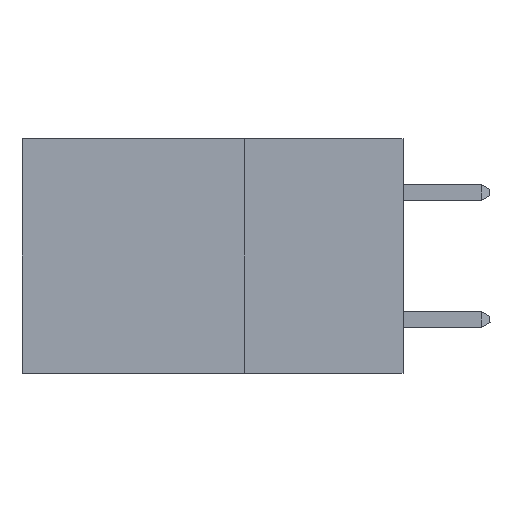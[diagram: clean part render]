
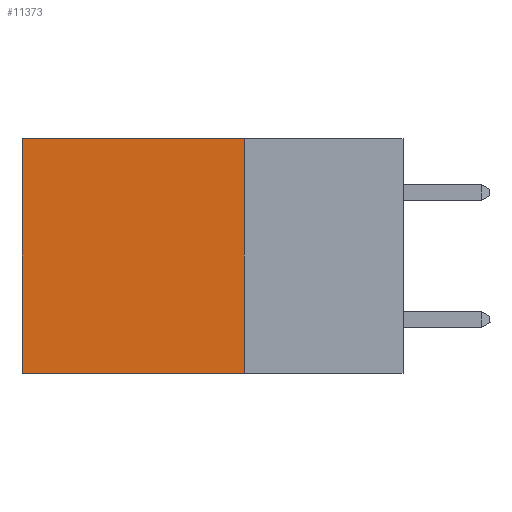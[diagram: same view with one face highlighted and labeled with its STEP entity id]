
A CAD part, left-side view. The second image highlights one B-rep face of the part: STEP entity #11373.
In plain terms, the highlighted planar face has unit normal (-1, 0, 0).
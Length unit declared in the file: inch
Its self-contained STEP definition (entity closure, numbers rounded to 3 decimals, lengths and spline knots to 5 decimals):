
#392 = CARTESIAN_POINT ( 'NONE',  ( 0.2875, 0.25, 0. ) ) ;
#699 = CARTESIAN_POINT ( 'NONE',  ( 0.2875, 0.25, -0.37 ) ) ;
#1184 = VECTOR ( 'NONE', #15054, 39.37008 ) ;
#1190 = CARTESIAN_POINT ( 'NONE',  ( 0.2875, 0.25, 0. ) ) ;
#1632 = LINE ( 'NONE', #13678, #1184 ) ;
#1925 = DIRECTION ( 'NONE',  ( 0., 0., -1. ) ) ;
#1986 = VECTOR ( 'NONE', #7826, 39.37008 ) ;
#1997 = CARTESIAN_POINT ( 'NONE',  ( 0.2875, 0.6, 0. ) ) ;
#2085 = CARTESIAN_POINT ( 'NONE',  ( 0.2875, 0.6, 0. ) ) ;
#2301 = EDGE_CURVE ( 'NONE', #9897, #3493, #14436, .T. ) ;
#2890 = VECTOR ( 'NONE', #3579, 39.37008 ) ;
#3493 = VERTEX_POINT ( 'NONE', #1997 ) ;
#3579 = DIRECTION ( 'NONE',  ( 0., 0., -1. ) ) ;
#3748 = ORIENTED_EDGE ( 'NONE', *, *, #7433, .F. ) ;
#3818 = ORIENTED_EDGE ( 'NONE', *, *, #7377, .T. ) ;
#4835 = VERTEX_POINT ( 'NONE', #8487 ) ;
#5856 = LINE ( 'NONE', #699, #13529 ) ;
#6582 = VERTEX_POINT ( 'NONE', #9240 ) ;
#7377 = EDGE_CURVE ( 'NONE', #3493, #4835, #17676, .T. ) ;
#7433 = EDGE_CURVE ( 'NONE', #6582, #4835, #5856, .T. ) ;
#7826 = DIRECTION ( 'NONE',  ( 0., 1., 0. ) ) ;
#7867 = CARTESIAN_POINT ( 'NONE',  ( 0.2875, 0.25, 0. ) ) ;
#8487 = CARTESIAN_POINT ( 'NONE',  ( 0.2875, 0.6, -0.37 ) ) ;
#8930 = EDGE_CURVE ( 'NONE', #9897, #6582, #1632, .T. ) ;
#9240 = CARTESIAN_POINT ( 'NONE',  ( 0.2875, 0.25, -0.37 ) ) ;
#9254 = PLANE ( 'NONE',  #13422 ) ;
#9710 = EDGE_LOOP ( 'NONE', ( #3818, #3748, #13375, #13694 ) ) ;
#9897 = VERTEX_POINT ( 'NONE', #1190 ) ;
#10704 = DIRECTION ( 'NONE',  ( 1., 0., 0. ) ) ;
#11373 = ADVANCED_FACE ( 'NONE', ( #15809 ), #9254, .F. ) ;
#12376 = DIRECTION ( 'NONE',  ( 0., 1., 0. ) ) ;
#13375 = ORIENTED_EDGE ( 'NONE', *, *, #8930, .F. ) ;
#13422 = AXIS2_PLACEMENT_3D ( 'NONE', #392, #10704, #1925 ) ;
#13529 = VECTOR ( 'NONE', #12376, 39.37008 ) ;
#13678 = CARTESIAN_POINT ( 'NONE',  ( 0.2875, 0.25, 0. ) ) ;
#13694 = ORIENTED_EDGE ( 'NONE', *, *, #2301, .T. ) ;
#14436 = LINE ( 'NONE', #7867, #1986 ) ;
#15054 = DIRECTION ( 'NONE',  ( 0., 0., -1. ) ) ;
#15809 = FACE_OUTER_BOUND ( 'NONE', #9710, .T. ) ;
#17676 = LINE ( 'NONE', #2085, #2890 ) ;
